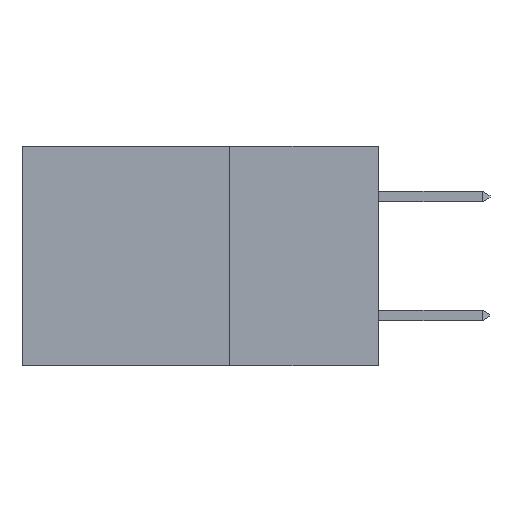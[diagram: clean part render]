
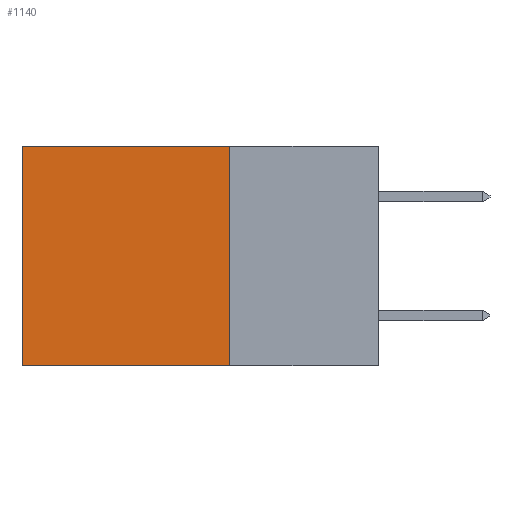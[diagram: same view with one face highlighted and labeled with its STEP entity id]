
A CAD part, left-side view. The second image highlights one B-rep face of the part: STEP entity #1140.
In plain terms, the highlighted planar face has unit normal (-1, 0, 0).
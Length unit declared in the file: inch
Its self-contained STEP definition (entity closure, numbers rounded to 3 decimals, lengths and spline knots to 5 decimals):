
#434 = EDGE_CURVE ( 'NONE', #11127, #10347, #5782, .T. ) ;
#1140 = ADVANCED_FACE ( 'NONE', ( #4665 ), #9577, .F. ) ;
#1377 = VECTOR ( 'NONE', #6830, 39.37008 ) ;
#1747 = CARTESIAN_POINT ( 'NONE',  ( 0.298, 0.6, -0.37 ) ) ;
#1776 = CARTESIAN_POINT ( 'NONE',  ( 0.298, 0.25, 0. ) ) ;
#2168 = EDGE_CURVE ( 'NONE', #6665, #11127, #11516, .T. ) ;
#2686 = ORIENTED_EDGE ( 'NONE', *, *, #434, .F. ) ;
#3727 = ORIENTED_EDGE ( 'NONE', *, *, #15041, .T. ) ;
#4433 = DIRECTION ( 'NONE',  ( 0., 0., -1. ) ) ;
#4665 = FACE_OUTER_BOUND ( 'NONE', #5517, .T. ) ;
#5156 = EDGE_CURVE ( 'NONE', #11781, #10347, #7169, .T. ) ;
#5517 = EDGE_LOOP ( 'NONE', ( #11467, #2686, #8598, #3727 ) ) ;
#5532 = CARTESIAN_POINT ( 'NONE',  ( 0.298, 0.6, 0. ) ) ;
#5782 = LINE ( 'NONE', #12715, #8630 ) ;
#5848 = AXIS2_PLACEMENT_3D ( 'NONE', #10825, #14489, #8482 ) ;
#6665 = VERTEX_POINT ( 'NONE', #13680 ) ;
#6830 = DIRECTION ( 'NONE',  ( 0., 0., -1. ) ) ;
#7169 = LINE ( 'NONE', #9234, #7540 ) ;
#7540 = VECTOR ( 'NONE', #4433, 39.37008 ) ;
#8482 = DIRECTION ( 'NONE',  ( 0., 0., -1. ) ) ;
#8598 = ORIENTED_EDGE ( 'NONE', *, *, #2168, .F. ) ;
#8630 = VECTOR ( 'NONE', #8786, 39.37008 ) ;
#8786 = DIRECTION ( 'NONE',  ( 0., 1., 0. ) ) ;
#9234 = CARTESIAN_POINT ( 'NONE',  ( 0.298, 0.6, 0. ) ) ;
#9257 = CARTESIAN_POINT ( 'NONE',  ( 0.298, 0.25, -0.37 ) ) ;
#9503 = LINE ( 'NONE', #1776, #11132 ) ;
#9577 = PLANE ( 'NONE',  #5848 ) ;
#9891 = CARTESIAN_POINT ( 'NONE',  ( 0.298, 0.25, 0. ) ) ;
#10347 = VERTEX_POINT ( 'NONE', #1747 ) ;
#10825 = CARTESIAN_POINT ( 'NONE',  ( 0.298, 0.25, 0. ) ) ;
#11127 = VERTEX_POINT ( 'NONE', #9257 ) ;
#11132 = VECTOR ( 'NONE', #11207, 39.37008 ) ;
#11207 = DIRECTION ( 'NONE',  ( 0., 1., 0. ) ) ;
#11467 = ORIENTED_EDGE ( 'NONE', *, *, #5156, .T. ) ;
#11516 = LINE ( 'NONE', #9891, #1377 ) ;
#11781 = VERTEX_POINT ( 'NONE', #5532 ) ;
#12715 = CARTESIAN_POINT ( 'NONE',  ( 0.298, 0.25, -0.37 ) ) ;
#13680 = CARTESIAN_POINT ( 'NONE',  ( 0.298, 0.25, 0. ) ) ;
#14489 = DIRECTION ( 'NONE',  ( 1., 0., 0. ) ) ;
#15041 = EDGE_CURVE ( 'NONE', #6665, #11781, #9503, .T. ) ;
